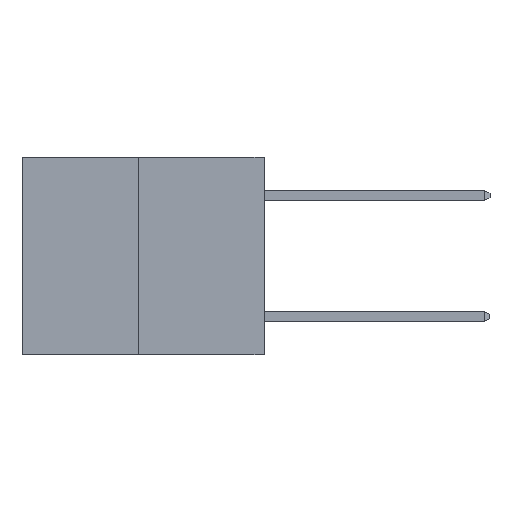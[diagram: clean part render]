
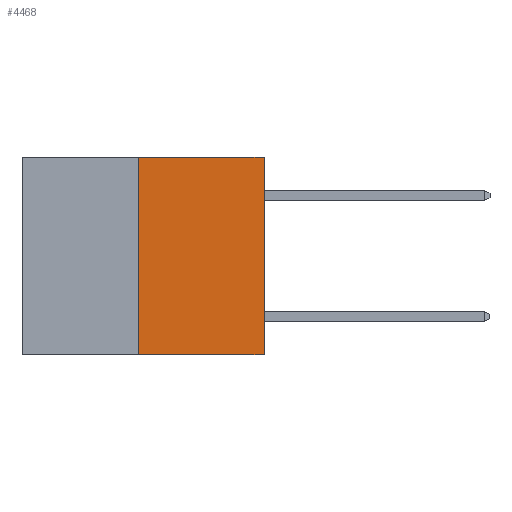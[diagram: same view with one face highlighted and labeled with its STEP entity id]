
A CAD part, left-side view. The second image highlights one B-rep face of the part: STEP entity #4468.
In plain terms, the highlighted planar face has unit normal (-1, 0, 0).
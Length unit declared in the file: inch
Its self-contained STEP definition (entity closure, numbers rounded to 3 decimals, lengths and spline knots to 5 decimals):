
#591 = CARTESIAN_POINT ( 'NONE',  ( 0., 0.6, -0.49 ) ) ;
#1214 = VERTEX_POINT ( 'NONE', #14798 ) ;
#1979 = VERTEX_POINT ( 'NONE', #12298 ) ;
#2721 = VECTOR ( 'NONE', #7643, 39.37008 ) ;
#2813 = VERTEX_POINT ( 'NONE', #7864 ) ;
#2861 = CARTESIAN_POINT ( 'NONE',  ( 0., 0.312, -0.49 ) ) ;
#2923 = LINE ( 'NONE', #591, #7486 ) ;
#2998 = VECTOR ( 'NONE', #4324, 39.37008 ) ;
#3200 = PLANE ( 'NONE',  #9569 ) ;
#4322 = ORIENTED_EDGE ( 'NONE', *, *, #9219, .T. ) ;
#4324 = DIRECTION ( 'NONE',  ( 0., 0., 1. ) ) ;
#4468 = ADVANCED_FACE ( 'NONE', ( #6195 ), #3200, .F. ) ;
#5001 = VECTOR ( 'NONE', #15027, 39.37008 ) ;
#5107 = ORIENTED_EDGE ( 'NONE', *, *, #5527, .F. ) ;
#5527 = EDGE_CURVE ( 'NONE', #9104, #2813, #13770, .T. ) ;
#5714 = CARTESIAN_POINT ( 'NONE',  ( 0., 0.6, 0. ) ) ;
#5772 = DIRECTION ( 'NONE',  ( 1., 0., 0. ) ) ;
#6195 = FACE_OUTER_BOUND ( 'NONE', #13148, .T. ) ;
#6423 = CARTESIAN_POINT ( 'NONE',  ( 0., 0.6, 0. ) ) ;
#6427 = CARTESIAN_POINT ( 'NONE',  ( 0., 0., 0. ) ) ;
#6620 = DIRECTION ( 'NONE',  ( 0., -1., 0. ) ) ;
#7486 = VECTOR ( 'NONE', #6620, 39.37008 ) ;
#7631 = ORIENTED_EDGE ( 'NONE', *, *, #13406, .F. ) ;
#7643 = DIRECTION ( 'NONE',  ( 0., 0., 1. ) ) ;
#7864 = CARTESIAN_POINT ( 'NONE',  ( 0., 0.312, 0. ) ) ;
#8716 = ORIENTED_EDGE ( 'NONE', *, *, #8765, .T. ) ;
#8765 = EDGE_CURVE ( 'NONE', #9104, #1214, #2923, .T. ) ;
#9104 = VERTEX_POINT ( 'NONE', #10942 ) ;
#9219 = EDGE_CURVE ( 'NONE', #1214, #1979, #13107, .T. ) ;
#9569 = AXIS2_PLACEMENT_3D ( 'NONE', #5714, #5772, #15484 ) ;
#10942 = CARTESIAN_POINT ( 'NONE',  ( 0., 0.312, -0.49 ) ) ;
#12298 = CARTESIAN_POINT ( 'NONE',  ( 0., 0., 0. ) ) ;
#13107 = LINE ( 'NONE', #6427, #2721 ) ;
#13148 = EDGE_LOOP ( 'NONE', ( #5107, #8716, #4322, #7631 ) ) ;
#13406 = EDGE_CURVE ( 'NONE', #2813, #1979, #15385, .T. ) ;
#13770 = LINE ( 'NONE', #2861, #2998 ) ;
#14798 = CARTESIAN_POINT ( 'NONE',  ( 0., 0., -0.49 ) ) ;
#15027 = DIRECTION ( 'NONE',  ( 0., -1., 0. ) ) ;
#15385 = LINE ( 'NONE', #6423, #5001 ) ;
#15484 = DIRECTION ( 'NONE',  ( 0., 0., -1. ) ) ;
